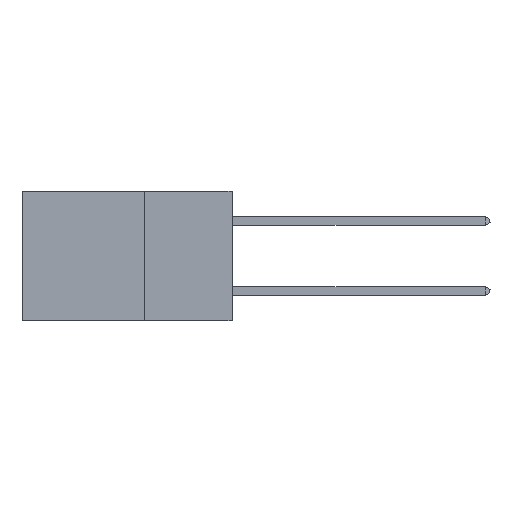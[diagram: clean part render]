
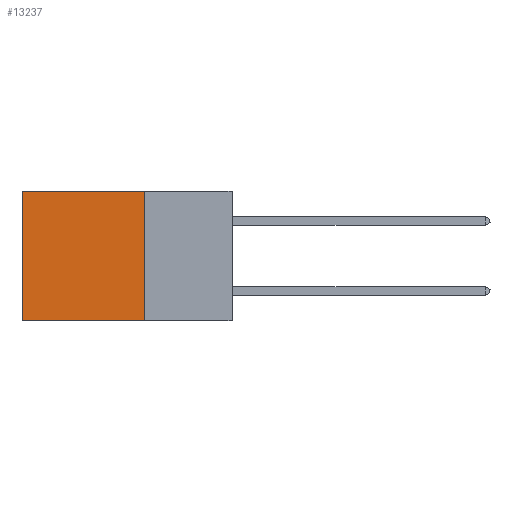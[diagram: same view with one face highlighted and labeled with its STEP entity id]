
A CAD part, left-side view. The second image highlights one B-rep face of the part: STEP entity #13237.
In plain terms, the highlighted planar face has unit normal (-1, 0, 0).
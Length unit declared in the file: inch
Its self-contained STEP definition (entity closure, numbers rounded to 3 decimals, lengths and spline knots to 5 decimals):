
#1299 = EDGE_LOOP ( 'NONE', ( #11590, #1987, #4362, #35778 ) ) ;
#1808 = VERTEX_POINT ( 'NONE', #9361 ) ;
#1987 = ORIENTED_EDGE ( 'NONE', *, *, #2630, .F. ) ;
#2222 = VECTOR ( 'NONE', #9537, 39.37008 ) ;
#2630 = EDGE_CURVE ( 'NONE', #1808, #26205, #6374, .T. ) ;
#2968 = EDGE_CURVE ( 'NONE', #36399, #1808, #15211, .T. ) ;
#3468 = PLANE ( 'NONE',  #4095 ) ;
#3721 = VECTOR ( 'NONE', #22452, 39.37008 ) ;
#3940 = LINE ( 'NONE', #24141, #2222 ) ;
#4095 = AXIS2_PLACEMENT_3D ( 'NONE', #9278, #29103, #6521 ) ;
#4362 = ORIENTED_EDGE ( 'NONE', *, *, #2968, .F. ) ;
#4576 = VECTOR ( 'NONE', #25609, 39.37008 ) ;
#5690 = CARTESIAN_POINT ( 'NONE',  ( 0.2875, 0.25, 0. ) ) ;
#6374 = LINE ( 'NONE', #10199, #3721 ) ;
#6521 = DIRECTION ( 'NONE',  ( 0., 0., -1. ) ) ;
#7404 = EDGE_CURVE ( 'NONE', #27164, #26205, #36479, .T. ) ;
#8802 = DIRECTION ( 'NONE',  ( 0., 0., -1. ) ) ;
#9204 = CARTESIAN_POINT ( 'NONE',  ( 0.2875, 0.6, -0.37 ) ) ;
#9278 = CARTESIAN_POINT ( 'NONE',  ( 0.2875, 0.25, 0. ) ) ;
#9361 = CARTESIAN_POINT ( 'NONE',  ( 0.2875, 0.25, -0.37 ) ) ;
#9537 = DIRECTION ( 'NONE',  ( 0., 1., 0. ) ) ;
#10199 = CARTESIAN_POINT ( 'NONE',  ( 0.2875, 0.25, -0.37 ) ) ;
#11590 = ORIENTED_EDGE ( 'NONE', *, *, #7404, .T. ) ;
#12602 = CARTESIAN_POINT ( 'NONE',  ( 0.2875, 0.25, 0. ) ) ;
#13237 = ADVANCED_FACE ( 'NONE', ( #15593 ), #3468, .F. ) ;
#15211 = LINE ( 'NONE', #5690, #4576 ) ;
#15593 = FACE_OUTER_BOUND ( 'NONE', #1299, .T. ) ;
#19189 = VECTOR ( 'NONE', #8802, 39.37008 ) ;
#20196 = CARTESIAN_POINT ( 'NONE',  ( 0.2875, 0.6, 0. ) ) ;
#21641 = EDGE_CURVE ( 'NONE', #36399, #27164, #3940, .T. ) ;
#22452 = DIRECTION ( 'NONE',  ( 0., 1., 0. ) ) ;
#24141 = CARTESIAN_POINT ( 'NONE',  ( 0.2875, 0.25, 0. ) ) ;
#25609 = DIRECTION ( 'NONE',  ( 0., 0., -1. ) ) ;
#26205 = VERTEX_POINT ( 'NONE', #9204 ) ;
#27164 = VERTEX_POINT ( 'NONE', #27242 ) ;
#27242 = CARTESIAN_POINT ( 'NONE',  ( 0.2875, 0.6, 0. ) ) ;
#29103 = DIRECTION ( 'NONE',  ( 1., 0., 0. ) ) ;
#35778 = ORIENTED_EDGE ( 'NONE', *, *, #21641, .T. ) ;
#36399 = VERTEX_POINT ( 'NONE', #12602 ) ;
#36479 = LINE ( 'NONE', #20196, #19189 ) ;
